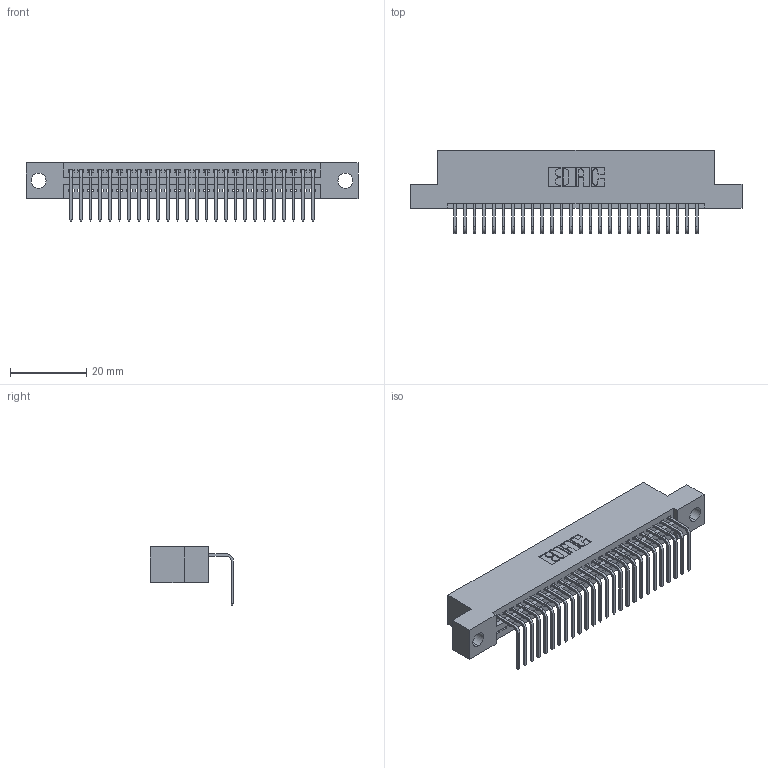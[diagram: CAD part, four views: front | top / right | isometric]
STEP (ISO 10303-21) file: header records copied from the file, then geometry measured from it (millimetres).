
FILE_DESCRIPTION (( 'STEP AP203' ), '1' );
FILE_NAME ('395-026-558-104.STEP', '2021-06-11T14:23:16', ( '' ), ( '' ), 'SwSTEP 2.0', 'SolidWorks 2020', '' );
FILE_SCHEMA (( 'CONFIG_CONTROL_DESIGN' ));
Length unit declared in the file: inch
Products named in the file (3): 395-026-558-104; 345-292-001_558 Tail - 2; 345 Part_Flush Mounting Lugs - 0.156 Dia-TI
Assembly tree (27 placements, depth 2):
  395-026-558-104
    345 Part_Flush Mounting Lugs - 0.156 Dia-TI
    345-292-001_558 Tail - 2  x26
Bounding box: 87.25 x 21.83 x 15.37 mm (x, y, z)
Volume: 8136.6 mm3; surface area: 10946.9 mm2
Topology: 27 solids, 27 shells, 1700 faces, 5109 edges, 3370 vertices
Faces by surface type: plane 1186, cylinder 514
Entity records: 22225 total; most frequent: CARTESIAN_POINT 3860, ORIENTED_EDGE 3818, DIRECTION 3393, EDGE_CURVE 1909, VECTOR 1673, LINE 1673, VERTEX_POINT 1270, AXIS2_PLACEMENT_3D 860
